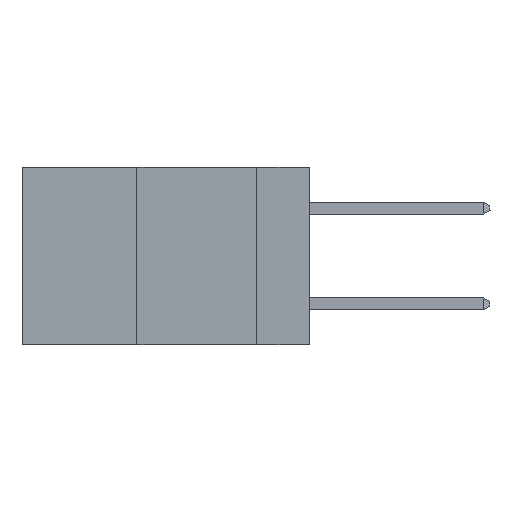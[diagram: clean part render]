
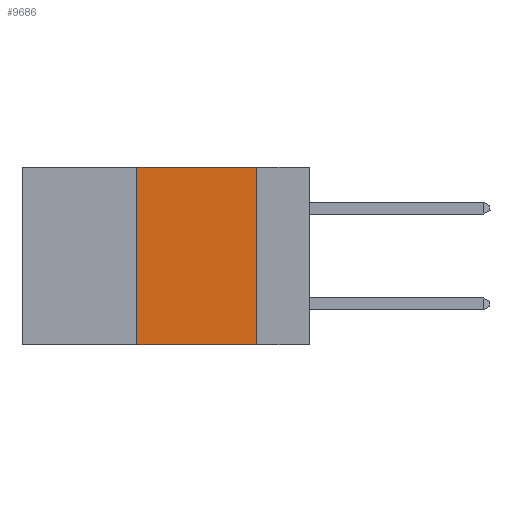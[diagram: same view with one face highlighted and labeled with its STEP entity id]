
A CAD part, left-side view. The second image highlights one B-rep face of the part: STEP entity #9686.
In plain terms, the highlighted planar face has unit normal (-1, 0, 0).
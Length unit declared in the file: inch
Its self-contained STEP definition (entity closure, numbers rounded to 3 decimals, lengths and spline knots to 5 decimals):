
#63 = CARTESIAN_POINT ( 'NONE',  ( 0., 0.36, 0. ) ) ;
#233 = LINE ( 'NONE', #4905, #6864 ) ;
#553 = ORIENTED_EDGE ( 'NONE', *, *, #5309, .F. ) ;
#875 = CARTESIAN_POINT ( 'NONE',  ( 0., 0.11, 0. ) ) ;
#1426 = LINE ( 'NONE', #4570, #7201 ) ;
#2441 = LINE ( 'NONE', #8756, #5789 ) ;
#2583 = EDGE_LOOP ( 'NONE', ( #3667, #7156, #553, #3101 ) ) ;
#3083 = VERTEX_POINT ( 'NONE', #4669 ) ;
#3101 = ORIENTED_EDGE ( 'NONE', *, *, #4024, .T. ) ;
#3667 = ORIENTED_EDGE ( 'NONE', *, *, #7151, .F. ) ;
#4024 = EDGE_CURVE ( 'NONE', #9186, #3083, #2441, .T. ) ;
#4036 = DIRECTION ( 'NONE',  ( 0., -1., 0. ) ) ;
#4482 = PLANE ( 'NONE',  #8066 ) ;
#4570 = CARTESIAN_POINT ( 'NONE',  ( 0., 0.11, 0. ) ) ;
#4669 = CARTESIAN_POINT ( 'NONE',  ( 0., 0.11, -0.37 ) ) ;
#4905 = CARTESIAN_POINT ( 'NONE',  ( 0., 0.36, 0. ) ) ;
#5309 = EDGE_CURVE ( 'NONE', #9186, #7031, #233, .T. ) ;
#5462 = DIRECTION ( 'NONE',  ( 0., 0., -1. ) ) ;
#5723 = DIRECTION ( 'NONE',  ( 0., 0., 1. ) ) ;
#5789 = VECTOR ( 'NONE', #4036, 39.37008 ) ;
#6168 = CARTESIAN_POINT ( 'NONE',  ( 0., 0.6, 0. ) ) ;
#6530 = DIRECTION ( 'NONE',  ( 0., -1., 0. ) ) ;
#6717 = EDGE_CURVE ( 'NONE', #7031, #7282, #10070, .T. ) ;
#6864 = VECTOR ( 'NONE', #5723, 39.37008 ) ;
#7031 = VERTEX_POINT ( 'NONE', #63 ) ;
#7151 = EDGE_CURVE ( 'NONE', #7282, #3083, #1426, .T. ) ;
#7156 = ORIENTED_EDGE ( 'NONE', *, *, #6717, .F. ) ;
#7195 = VECTOR ( 'NONE', #6530, 39.37008 ) ;
#7201 = VECTOR ( 'NONE', #7698, 39.37008 ) ;
#7282 = VERTEX_POINT ( 'NONE', #875 ) ;
#7698 = DIRECTION ( 'NONE',  ( 0., 0., -1. ) ) ;
#7764 = CARTESIAN_POINT ( 'NONE',  ( 0., 0.6, 0. ) ) ;
#8066 = AXIS2_PLACEMENT_3D ( 'NONE', #7764, #8377, #5462 ) ;
#8377 = DIRECTION ( 'NONE',  ( 1., 0., 0. ) ) ;
#8537 = FACE_OUTER_BOUND ( 'NONE', #2583, .T. ) ;
#8756 = CARTESIAN_POINT ( 'NONE',  ( 0., 0.6, -0.37 ) ) ;
#8967 = CARTESIAN_POINT ( 'NONE',  ( 0., 0.36, -0.37 ) ) ;
#9186 = VERTEX_POINT ( 'NONE', #8967 ) ;
#9686 = ADVANCED_FACE ( 'NONE', ( #8537 ), #4482, .F. ) ;
#10070 = LINE ( 'NONE', #6168, #7195 ) ;
